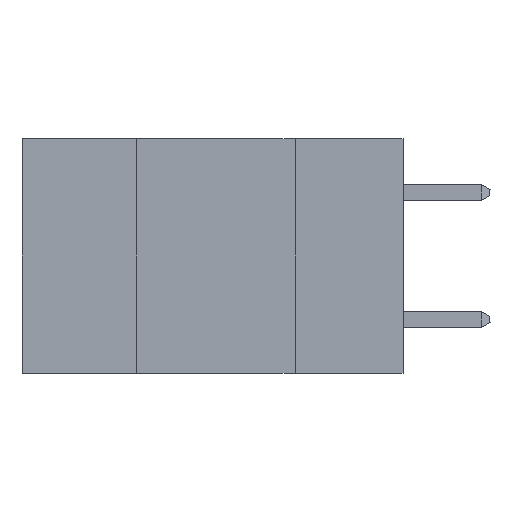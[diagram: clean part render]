
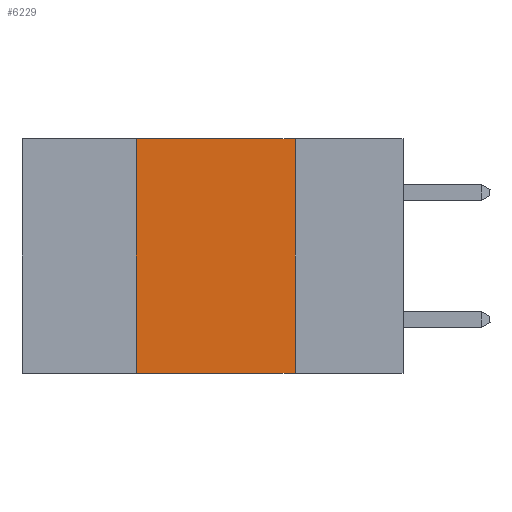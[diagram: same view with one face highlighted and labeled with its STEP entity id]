
A CAD part, left-side view. The second image highlights one B-rep face of the part: STEP entity #6229.
In plain terms, the highlighted planar face has unit normal (-1, 0, 0).
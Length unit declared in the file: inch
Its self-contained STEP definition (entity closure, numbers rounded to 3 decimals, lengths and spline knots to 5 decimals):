
#153 = DIRECTION ( 'NONE',  ( 0., -1., 0. ) ) ;
#590 = FACE_OUTER_BOUND ( 'NONE', #4504, .T. ) ;
#596 = EDGE_CURVE ( 'NONE', #15192, #3906, #1307, .T. ) ;
#627 = ORIENTED_EDGE ( 'NONE', *, *, #15122, .F. ) ;
#719 = CARTESIAN_POINT ( 'NONE',  ( 0., 0.17, -0.37 ) ) ;
#1307 = LINE ( 'NONE', #12999, #11064 ) ;
#1369 = VECTOR ( 'NONE', #7459, 39.37008 ) ;
#1446 = CARTESIAN_POINT ( 'NONE',  ( 0., 0.6, 0. ) ) ;
#1802 = CARTESIAN_POINT ( 'NONE',  ( 0., 0.6, 0. ) ) ;
#1903 = VERTEX_POINT ( 'NONE', #9905 ) ;
#3030 = ORIENTED_EDGE ( 'NONE', *, *, #6164, .F. ) ;
#3222 = CARTESIAN_POINT ( 'NONE',  ( 0., 0.6, -0.37 ) ) ;
#3906 = VERTEX_POINT ( 'NONE', #719 ) ;
#4354 = EDGE_CURVE ( 'NONE', #8168, #3906, #8246, .T. ) ;
#4404 = PLANE ( 'NONE',  #12778 ) ;
#4504 = EDGE_LOOP ( 'NONE', ( #12405, #3030, #627, #10374 ) ) ;
#4506 = LINE ( 'NONE', #1446, #13864 ) ;
#4950 = DIRECTION ( 'NONE',  ( 1., 0., 0. ) ) ;
#6164 = EDGE_CURVE ( 'NONE', #1903, #15192, #4506, .T. ) ;
#6229 = ADVANCED_FACE ( 'NONE', ( #590 ), #4404, .F. ) ;
#6245 = CARTESIAN_POINT ( 'NONE',  ( 0., 0.17, 0. ) ) ;
#7459 = DIRECTION ( 'NONE',  ( 0., 0., 1. ) ) ;
#8168 = VERTEX_POINT ( 'NONE', #8805 ) ;
#8246 = LINE ( 'NONE', #3222, #13896 ) ;
#8805 = CARTESIAN_POINT ( 'NONE',  ( 0., 0.42, -0.37 ) ) ;
#9905 = CARTESIAN_POINT ( 'NONE',  ( 0., 0.42, 0. ) ) ;
#10050 = DIRECTION ( 'NONE',  ( 0., -1., 0. ) ) ;
#10374 = ORIENTED_EDGE ( 'NONE', *, *, #4354, .T. ) ;
#10843 = DIRECTION ( 'NONE',  ( 0., 0., -1. ) ) ;
#11064 = VECTOR ( 'NONE', #12797, 39.37008 ) ;
#12405 = ORIENTED_EDGE ( 'NONE', *, *, #596, .F. ) ;
#12778 = AXIS2_PLACEMENT_3D ( 'NONE', #1802, #4950, #10843 ) ;
#12797 = DIRECTION ( 'NONE',  ( 0., 0., -1. ) ) ;
#12999 = CARTESIAN_POINT ( 'NONE',  ( 0., 0.17, 0. ) ) ;
#13864 = VECTOR ( 'NONE', #10050, 39.37008 ) ;
#13896 = VECTOR ( 'NONE', #153, 39.37008 ) ;
#13900 = LINE ( 'NONE', #14682, #1369 ) ;
#14682 = CARTESIAN_POINT ( 'NONE',  ( 0., 0.42, 0. ) ) ;
#15122 = EDGE_CURVE ( 'NONE', #8168, #1903, #13900, .T. ) ;
#15192 = VERTEX_POINT ( 'NONE', #6245 ) ;
